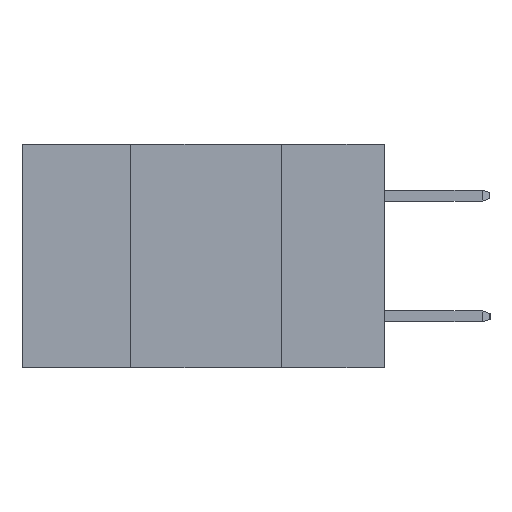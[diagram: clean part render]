
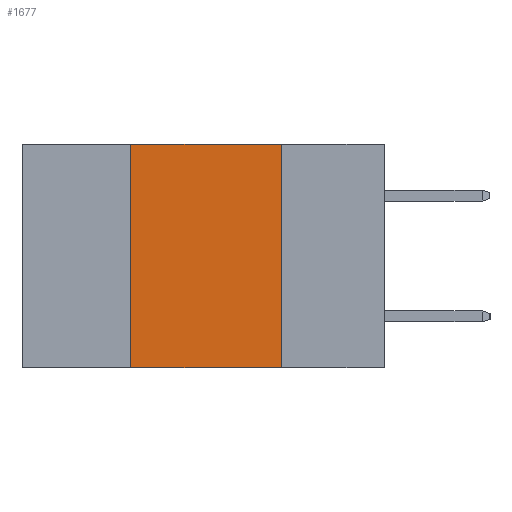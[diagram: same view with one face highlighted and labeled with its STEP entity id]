
A CAD part, left-side view. The second image highlights one B-rep face of the part: STEP entity #1677.
In plain terms, the highlighted planar face has unit normal (-1, 0, 0).
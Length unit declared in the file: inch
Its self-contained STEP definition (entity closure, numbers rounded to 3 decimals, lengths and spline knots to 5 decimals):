
#95 = DIRECTION ( 'NONE',  ( 0., 0., 1. ) ) ;
#644 = VERTEX_POINT ( 'NONE', #4454 ) ;
#798 = DIRECTION ( 'NONE',  ( 0., 0., -1. ) ) ;
#943 = EDGE_CURVE ( 'NONE', #10197, #6799, #5256, .T. ) ;
#1279 = VECTOR ( 'NONE', #3231, 39.37008 ) ;
#1677 = ADVANCED_FACE ( 'NONE', ( #9895 ), #5477, .F. ) ;
#2538 = CARTESIAN_POINT ( 'NONE',  ( 0., 0.17, -0.37 ) ) ;
#3231 = DIRECTION ( 'NONE',  ( 0., -1., 0. ) ) ;
#3372 = VECTOR ( 'NONE', #798, 39.37008 ) ;
#3382 = ORIENTED_EDGE ( 'NONE', *, *, #943, .T. ) ;
#3435 = EDGE_CURVE ( 'NONE', #644, #6799, #8173, .T. ) ;
#3515 = DIRECTION ( 'NONE',  ( 0., -1., 0. ) ) ;
#3552 = CARTESIAN_POINT ( 'NONE',  ( 0., 0.42, -0.37 ) ) ;
#3865 = LINE ( 'NONE', #3552, #9829 ) ;
#4042 = LINE ( 'NONE', #8088, #1279 ) ;
#4267 = ORIENTED_EDGE ( 'NONE', *, *, #3435, .F. ) ;
#4454 = CARTESIAN_POINT ( 'NONE',  ( 0., 0.17, 0. ) ) ;
#4519 = CARTESIAN_POINT ( 'NONE',  ( 0., 0.42, -0.37 ) ) ;
#4526 = ORIENTED_EDGE ( 'NONE', *, *, #9156, .F. ) ;
#4668 = CARTESIAN_POINT ( 'NONE',  ( 0., 0.6, -0.37 ) ) ;
#4730 = DIRECTION ( 'NONE',  ( 0., 0., -1. ) ) ;
#5118 = DIRECTION ( 'NONE',  ( 1., 0., 0. ) ) ;
#5199 = CARTESIAN_POINT ( 'NONE',  ( 0., 0.6, 0. ) ) ;
#5256 = LINE ( 'NONE', #4668, #8891 ) ;
#5382 = CARTESIAN_POINT ( 'NONE',  ( 0., 0.17, -0.37 ) ) ;
#5477 = PLANE ( 'NONE',  #8600 ) ;
#6243 = VERTEX_POINT ( 'NONE', #9837 ) ;
#6467 = EDGE_CURVE ( 'NONE', #6243, #644, #4042, .T. ) ;
#6799 = VERTEX_POINT ( 'NONE', #5382 ) ;
#8088 = CARTESIAN_POINT ( 'NONE',  ( 0., 0.6, 0. ) ) ;
#8173 = LINE ( 'NONE', #2538, #3372 ) ;
#8600 = AXIS2_PLACEMENT_3D ( 'NONE', #5199, #5118, #4730 ) ;
#8891 = VECTOR ( 'NONE', #3515, 39.37008 ) ;
#9127 = EDGE_LOOP ( 'NONE', ( #4267, #10433, #4526, #3382 ) ) ;
#9156 = EDGE_CURVE ( 'NONE', #10197, #6243, #3865, .T. ) ;
#9829 = VECTOR ( 'NONE', #95, 39.37008 ) ;
#9837 = CARTESIAN_POINT ( 'NONE',  ( 0., 0.42, 0. ) ) ;
#9895 = FACE_OUTER_BOUND ( 'NONE', #9127, .T. ) ;
#10197 = VERTEX_POINT ( 'NONE', #4519 ) ;
#10433 = ORIENTED_EDGE ( 'NONE', *, *, #6467, .F. ) ;
